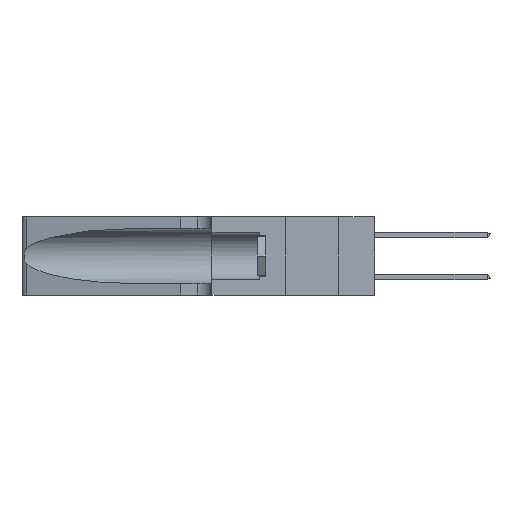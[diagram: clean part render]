
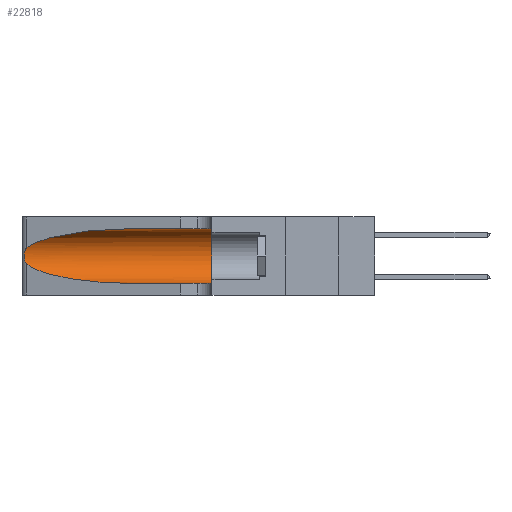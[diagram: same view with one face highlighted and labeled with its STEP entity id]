
A CAD part, left-side view. The second image highlights one B-rep face of the part: STEP entity #22818.
In plain terms, the highlighted cylindrical face has radius 3.308 mm (diameter 6.617 mm), a partial arc.
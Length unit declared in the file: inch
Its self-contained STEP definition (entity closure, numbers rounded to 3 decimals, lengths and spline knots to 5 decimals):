
#395 =( BOUNDED_CURVE ( )  B_SPLINE_CURVE ( 3, ( #9104, #7269, #20145, #21952 ),
 .UNSPECIFIED., .F., .T. ) 
 B_SPLINE_CURVE_WITH_KNOTS ( ( 4, 4 ),
 ( 3.44316, 4.71239 ),
 .UNSPECIFIED. ) 
 CURVE ( )  GEOMETRIC_REPRESENTATION_ITEM ( )  RATIONAL_B_SPLINE_CURVE ( ( 1., 0.87, 0.87, 1. ) ) 
 REPRESENTATION_ITEM ( '' )  );
#512 = CARTESIAN_POINT ( 'NONE',  ( 0.18966, 0.96281, 0.31525 ) ) ;
#1296 = ORIENTED_EDGE ( 'NONE', *, *, #13297, .F. ) ;
#2046 = ORIENTED_EDGE ( 'NONE', *, *, #3499, .F. ) ;
#2532 = CARTESIAN_POINT ( 'NONE',  ( 0.25487, 1.22718, 0.22369 ) ) ;
#2730 = EDGE_CURVE ( 'NONE', #12398, #7301, #395, .T. ) ;
#2878 = CARTESIAN_POINT ( 'NONE',  ( 0.25787, 1.23484, 0.2124 ) ) ;
#3151 = CYLINDRICAL_SURFACE ( 'NONE', #3273, 0.13025 ) ;
#3273 = AXIS2_PLACEMENT_3D ( 'NONE', #9609, #22421, #5868 ) ;
#3499 = EDGE_CURVE ( 'NONE', #4685, #22685, #15294, .T. ) ;
#3641 = VERTEX_POINT ( 'NONE', #22464 ) ;
#3653 = AXIS2_PLACEMENT_3D ( 'NONE', #20352, #9309, #22146 ) ;
#4314 = CARTESIAN_POINT ( 'NONE',  ( 0.1305, 1.61858, 0.31525 ) ) ;
#4593 = EDGE_CURVE ( 'NONE', #7301, #22685, #8526, .T. ) ;
#4685 = VERTEX_POINT ( 'NONE', #12379 ) ;
#4834 = CARTESIAN_POINT ( 'NONE',  ( 0.26018, 1.23835, 0.19895 ) ) ;
#5084 = VERTEX_POINT ( 'NONE', #15249 ) ;
#5868 = DIRECTION ( 'NONE',  ( 0., 0., -1. ) ) ;
#6690 = CARTESIAN_POINT ( 'NONE',  ( 0.25555, 1.22994, 0.2215 ) ) ;
#6772 = CARTESIAN_POINT ( 'NONE',  ( 0.26075, 1.23896, 0.178 ) ) ;
#7269 = CARTESIAN_POINT ( 'NONE',  ( 0.2373, 1.15595, 0.08982 ) ) ;
#7301 = VERTEX_POINT ( 'NONE', #21360 ) ;
#8225 = ORIENTED_EDGE ( 'NONE', *, *, #11229, .T. ) ;
#8526 = LINE ( 'NONE', #17482, #22574 ) ;
#8632 = CARTESIAN_POINT ( 'NONE',  ( 0.25856, 1.23593, 0.16098 ) ) ;
#9056 = CARTESIAN_POINT ( 'NONE',  ( 0.25487, 1.22718, 0.14631 ) ) ;
#9104 = CARTESIAN_POINT ( 'NONE',  ( 0.25487, 1.22718, 0.14631 ) ) ;
#9309 = DIRECTION ( 'NONE',  ( 0., 1., 0. ) ) ;
#9609 = CARTESIAN_POINT ( 'NONE',  ( 0.1305, 1.61858, 0.185 ) ) ;
#9704 = ORIENTED_EDGE ( 'NONE', *, *, #11121, .T. ) ;
#10431 = CARTESIAN_POINT ( 'NONE',  ( 0.25487, 1.22718, 0.22369 ) ) ;
#10523 = CARTESIAN_POINT ( 'NONE',  ( 0.25639, 1.23186, 0.15144 ) ) ;
#10880 = LINE ( 'NONE', #4314, #20064 ) ;
#11103 = CARTESIAN_POINT ( 'NONE',  ( 0.1305, 0.35, 0.05475 ) ) ;
#11121 = EDGE_CURVE ( 'NONE', #3641, #5084, #19540, .T. ) ;
#11229 = EDGE_CURVE ( 'NONE', #5084, #12398, #15287, .T. ) ;
#11977 = CARTESIAN_POINT ( 'NONE',  ( 0.1305, 0.72297, 0.31525 ) ) ;
#12378 = CARTESIAN_POINT ( 'NONE',  ( 0.25487, 1.22718, 0.14631 ) ) ;
#12379 = CARTESIAN_POINT ( 'NONE',  ( 0.1305, 0.35, 0.31525 ) ) ;
#12398 = VERTEX_POINT ( 'NONE', #9056 ) ;
#13297 = EDGE_CURVE ( 'NONE', #3641, #4685, #10880, .T. ) ;
#13826 = CARTESIAN_POINT ( 'NONE',  ( 0.2373, 1.15595, 0.28018 ) ) ;
#14160 = CARTESIAN_POINT ( 'NONE',  ( 0.25639, 1.23184, 0.21858 ) ) ;
#15249 = CARTESIAN_POINT ( 'NONE',  ( 0.25487, 1.22718, 0.22369 ) ) ;
#15287 = B_SPLINE_CURVE_WITH_KNOTS ( 'NONE', 3,
 ( #10431, #6690, #14160, #2878, #15996, #4834, #17810, #6772, #19669, #8632, #21483, #10523, #23314, #12378 ),
 .UNSPECIFIED., .F., .F.,
 ( 4, 2, 2, 2, 2, 2, 4 ),
 ( 0., 0.00027, 0.00053, 0.00107, 0.0016, 0.00187, 0.00214 ),
 .UNSPECIFIED. ) ;
#15294 = CIRCLE ( 'NONE', #3653, 0.13025 ) ;
#15783 = ORIENTED_EDGE ( 'NONE', *, *, #4593, .T. ) ;
#15996 = CARTESIAN_POINT ( 'NONE',  ( 0.25854, 1.2359, 0.20912 ) ) ;
#17482 = CARTESIAN_POINT ( 'NONE',  ( 0.1305, 1.61858, 0.05475 ) ) ;
#17810 = CARTESIAN_POINT ( 'NONE',  ( 0.26075, 1.23896, 0.19203 ) ) ;
#18023 = FACE_OUTER_BOUND ( 'NONE', #19720, .T. ) ;
#19170 = DIRECTION ( 'NONE',  ( 0., -1., 0. ) ) ;
#19429 = DIRECTION ( 'NONE',  ( 0., -1., 0. ) ) ;
#19540 =( BOUNDED_CURVE ( )  B_SPLINE_CURVE ( 3, ( #11977, #512, #13826, #2532 ),
 .UNSPECIFIED., .F., .T. ) 
 B_SPLINE_CURVE_WITH_KNOTS ( ( 4, 4 ),
 ( 1.5708, 2.84003 ),
 .UNSPECIFIED. ) 
 CURVE ( )  GEOMETRIC_REPRESENTATION_ITEM ( )  RATIONAL_B_SPLINE_CURVE ( ( 1., 0.87, 0.87, 1. ) ) 
 REPRESENTATION_ITEM ( '' )  );
#19669 = CARTESIAN_POINT ( 'NONE',  ( 0.26017, 1.23833, 0.17102 ) ) ;
#19720 = EDGE_LOOP ( 'NONE', ( #9704, #8225, #23792, #15783, #2046, #1296 ) ) ;
#20064 = VECTOR ( 'NONE', #19170, 39.37008 ) ;
#20145 = CARTESIAN_POINT ( 'NONE',  ( 0.18966, 0.96281, 0.05475 ) ) ;
#20352 = CARTESIAN_POINT ( 'NONE',  ( 0.1305, 0.35, 0.185 ) ) ;
#21360 = CARTESIAN_POINT ( 'NONE',  ( 0.1305, 0.72297, 0.05475 ) ) ;
#21483 = CARTESIAN_POINT ( 'NONE',  ( 0.25789, 1.23486, 0.15765 ) ) ;
#21952 = CARTESIAN_POINT ( 'NONE',  ( 0.1305, 0.72297, 0.05475 ) ) ;
#22146 = DIRECTION ( 'NONE',  ( 0., 0., 1. ) ) ;
#22421 = DIRECTION ( 'NONE',  ( 0., -1., 0. ) ) ;
#22464 = CARTESIAN_POINT ( 'NONE',  ( 0.1305, 0.72297, 0.31525 ) ) ;
#22574 = VECTOR ( 'NONE', #19429, 39.37008 ) ;
#22685 = VERTEX_POINT ( 'NONE', #11103 ) ;
#22818 = ADVANCED_FACE ( 'NONE', ( #18023 ), #3151, .F. ) ;
#23314 = CARTESIAN_POINT ( 'NONE',  ( 0.25555, 1.22993, 0.14849 ) ) ;
#23792 = ORIENTED_EDGE ( 'NONE', *, *, #2730, .T. ) ;
